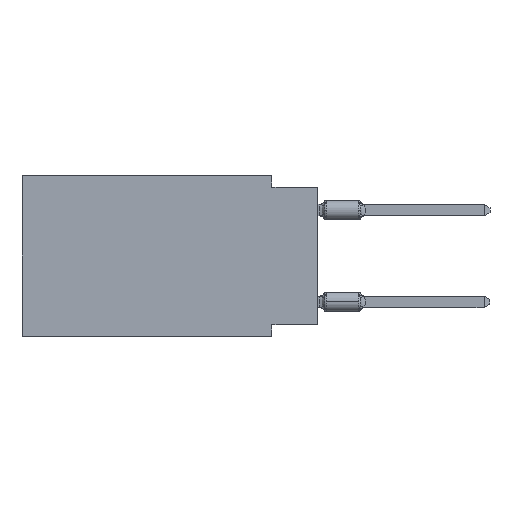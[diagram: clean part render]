
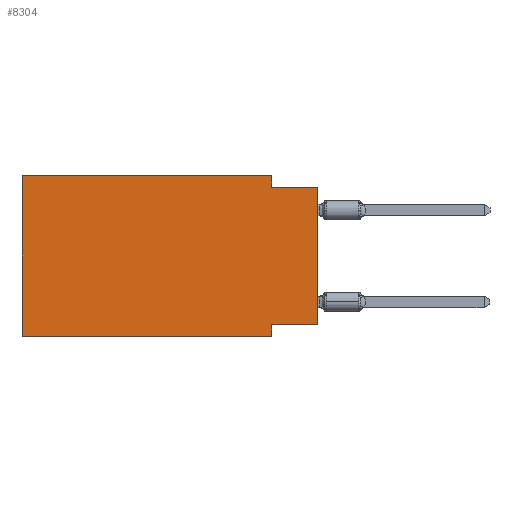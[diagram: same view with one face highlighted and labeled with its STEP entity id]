
A CAD part, left-side view. The second image highlights one B-rep face of the part: STEP entity #8304.
In plain terms, the highlighted planar face has unit normal (-1, 0, 0).
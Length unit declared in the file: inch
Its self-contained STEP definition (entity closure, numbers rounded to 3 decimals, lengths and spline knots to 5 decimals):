
#526 = DIRECTION ( 'NONE',  ( 0., -1., 0. ) ) ;
#690 = ORIENTED_EDGE ( 'NONE', *, *, #15021, .F. ) ;
#1340 = CARTESIAN_POINT ( 'NONE',  ( 0., 0.645, 0. ) ) ;
#1620 = VERTEX_POINT ( 'NONE', #1792 ) ;
#1792 = CARTESIAN_POINT ( 'NONE',  ( 0., 0.1, -0.325 ) ) ;
#2244 = CARTESIAN_POINT ( 'NONE',  ( 0., 0.1, -0.35 ) ) ;
#2273 = ORIENTED_EDGE ( 'NONE', *, *, #13949, .F. ) ;
#2911 = EDGE_LOOP ( 'NONE', ( #19591, #16837, #4355, #14300, #690, #17007, #5848, #2273 ) ) ;
#3165 = LINE ( 'NONE', #15472, #6294 ) ;
#3779 = EDGE_CURVE ( 'NONE', #9536, #19073, #12841, .T. ) ;
#4355 = ORIENTED_EDGE ( 'NONE', *, *, #18749, .F. ) ;
#4770 = DIRECTION ( 'NONE',  ( 0., -1., 0. ) ) ;
#4886 = DIRECTION ( 'NONE',  ( 1., 0., 0. ) ) ;
#5210 = CARTESIAN_POINT ( 'NONE',  ( 0., 0.645, 0. ) ) ;
#5642 = VERTEX_POINT ( 'NONE', #17671 ) ;
#5753 = VECTOR ( 'NONE', #7498, 39.37008 ) ;
#5848 = ORIENTED_EDGE ( 'NONE', *, *, #10545, .F. ) ;
#5876 = CARTESIAN_POINT ( 'NONE',  ( 0., 0.645, -0.35 ) ) ;
#5969 = CARTESIAN_POINT ( 'NONE',  ( 0., 0., -0.325 ) ) ;
#6294 = VECTOR ( 'NONE', #4770, 39.37008 ) ;
#6348 = EDGE_CURVE ( 'NONE', #12024, #5642, #15184, .T. ) ;
#7247 = VERTEX_POINT ( 'NONE', #17817 ) ;
#7498 = DIRECTION ( 'NONE',  ( 0., -1., 0. ) ) ;
#7569 = VECTOR ( 'NONE', #19228, 39.37008 ) ;
#8210 = CARTESIAN_POINT ( 'NONE',  ( 0., 0., -0.025 ) ) ;
#8304 = ADVANCED_FACE ( 'NONE', ( #13958 ), #12550, .F. ) ;
#8636 = VECTOR ( 'NONE', #9008, 39.37008 ) ;
#9008 = DIRECTION ( 'NONE',  ( 0., 1., 0. ) ) ;
#9536 = VERTEX_POINT ( 'NONE', #19151 ) ;
#9568 = VECTOR ( 'NONE', #526, 39.37008 ) ;
#10545 = EDGE_CURVE ( 'NONE', #1620, #7247, #13129, .T. ) ;
#11047 = DIRECTION ( 'NONE',  ( 0., 0., -1. ) ) ;
#11127 = DIRECTION ( 'NONE',  ( 0., 0., -1. ) ) ;
#12024 = VERTEX_POINT ( 'NONE', #13463 ) ;
#12550 = PLANE ( 'NONE',  #15063 ) ;
#12554 = CARTESIAN_POINT ( 'NONE',  ( 0., 0., -0.025 ) ) ;
#12841 = LINE ( 'NONE', #8210, #9568 ) ;
#13129 = LINE ( 'NONE', #2244, #14267 ) ;
#13463 = CARTESIAN_POINT ( 'NONE',  ( 0., 0.645, 0. ) ) ;
#13949 = EDGE_CURVE ( 'NONE', #18133, #1620, #19792, .T. ) ;
#13958 = FACE_OUTER_BOUND ( 'NONE', #2911, .T. ) ;
#14141 = LINE ( 'NONE', #18794, #19320 ) ;
#14267 = VECTOR ( 'NONE', #14557, 39.37008 ) ;
#14300 = ORIENTED_EDGE ( 'NONE', *, *, #6348, .F. ) ;
#14498 = LINE ( 'NONE', #5210, #7569 ) ;
#14557 = DIRECTION ( 'NONE',  ( 0., 0., -1. ) ) ;
#15021 = EDGE_CURVE ( 'NONE', #18605, #12024, #14498, .T. ) ;
#15063 = AXIS2_PLACEMENT_3D ( 'NONE', #18719, #4886, #11047 ) ;
#15184 = LINE ( 'NONE', #1340, #5753 ) ;
#15472 = CARTESIAN_POINT ( 'NONE',  ( 0., 0.645, -0.35 ) ) ;
#15549 = DIRECTION ( 'NONE',  ( 0., 0., 1. ) ) ;
#15956 = LINE ( 'NONE', #19062, #19492 ) ;
#16204 = EDGE_CURVE ( 'NONE', #18605, #7247, #3165, .T. ) ;
#16412 = CARTESIAN_POINT ( 'NONE',  ( 0., 0., -0.325 ) ) ;
#16694 = EDGE_CURVE ( 'NONE', #18133, #19073, #15956, .T. ) ;
#16837 = ORIENTED_EDGE ( 'NONE', *, *, #3779, .F. ) ;
#17007 = ORIENTED_EDGE ( 'NONE', *, *, #16204, .T. ) ;
#17671 = CARTESIAN_POINT ( 'NONE',  ( 0., 0.1, 0. ) ) ;
#17817 = CARTESIAN_POINT ( 'NONE',  ( 0., 0.1, -0.35 ) ) ;
#18133 = VERTEX_POINT ( 'NONE', #16412 ) ;
#18605 = VERTEX_POINT ( 'NONE', #5876 ) ;
#18719 = CARTESIAN_POINT ( 'NONE',  ( 0., 0.645, 0. ) ) ;
#18749 = EDGE_CURVE ( 'NONE', #5642, #9536, #14141, .T. ) ;
#18794 = CARTESIAN_POINT ( 'NONE',  ( 0., 0.1, 0. ) ) ;
#19062 = CARTESIAN_POINT ( 'NONE',  ( 0., 0., 0. ) ) ;
#19073 = VERTEX_POINT ( 'NONE', #12554 ) ;
#19151 = CARTESIAN_POINT ( 'NONE',  ( 0., 0.1, -0.025 ) ) ;
#19228 = DIRECTION ( 'NONE',  ( 0., 0., 1. ) ) ;
#19320 = VECTOR ( 'NONE', #11127, 39.37008 ) ;
#19492 = VECTOR ( 'NONE', #15549, 39.37008 ) ;
#19591 = ORIENTED_EDGE ( 'NONE', *, *, #16694, .T. ) ;
#19792 = LINE ( 'NONE', #5969, #8636 ) ;
